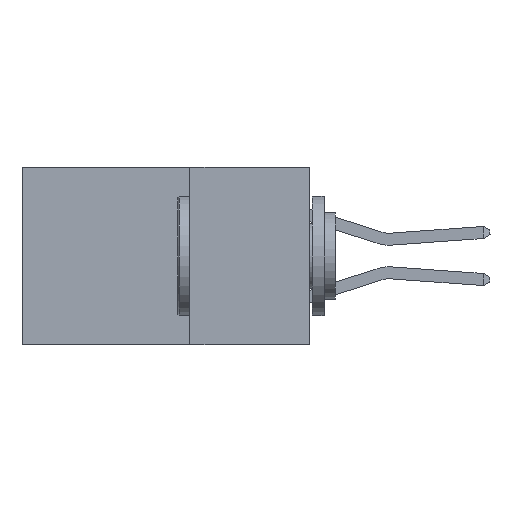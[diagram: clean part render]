
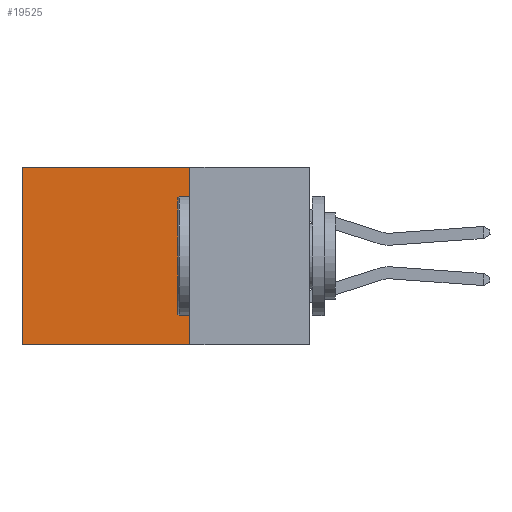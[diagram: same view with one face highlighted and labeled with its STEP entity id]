
A CAD part, left-side view. The second image highlights one B-rep face of the part: STEP entity #19525.
In plain terms, the highlighted planar face has unit normal (-1, 0, 0).
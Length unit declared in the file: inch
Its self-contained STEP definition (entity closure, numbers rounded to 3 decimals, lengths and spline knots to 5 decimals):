
#249 = VERTEX_POINT ( 'NONE', #23125 ) ;
#716 = CARTESIAN_POINT ( 'NONE',  ( 0.2615, 0.6, -0.37 ) ) ;
#1182 = LINE ( 'NONE', #8395, #9789 ) ;
#1190 = CARTESIAN_POINT ( 'NONE',  ( 0.2615, 0.25, -0.37 ) ) ;
#1338 = FACE_OUTER_BOUND ( 'NONE', #1644, .T. ) ;
#1423 = DIRECTION ( 'NONE',  ( 0., 0., -1. ) ) ;
#1644 = EDGE_LOOP ( 'NONE', ( #18930, #4151, #7641, #22586 ) ) ;
#3120 = LINE ( 'NONE', #13941, #11418 ) ;
#3147 = CARTESIAN_POINT ( 'NONE',  ( 0.2615, 0.25, 0. ) ) ;
#4151 = ORIENTED_EDGE ( 'NONE', *, *, #6804, .F. ) ;
#4480 = CARTESIAN_POINT ( 'NONE',  ( 0.2615, 0.6, 0. ) ) ;
#6804 = EDGE_CURVE ( 'NONE', #10332, #18355, #3120, .T. ) ;
#6813 = LINE ( 'NONE', #3147, #8588 ) ;
#7641 = ORIENTED_EDGE ( 'NONE', *, *, #16873, .F. ) ;
#8043 = AXIS2_PLACEMENT_3D ( 'NONE', #8551, #15694, #13925 ) ;
#8395 = CARTESIAN_POINT ( 'NONE',  ( 0.2615, 0.25, -0.37 ) ) ;
#8551 = CARTESIAN_POINT ( 'NONE',  ( 0.2615, 0.25, -0.37 ) ) ;
#8588 = VECTOR ( 'NONE', #19231, 39.37008 ) ;
#9208 = VECTOR ( 'NONE', #12108, 39.37008 ) ;
#9337 = VERTEX_POINT ( 'NONE', #4480 ) ;
#9789 = VECTOR ( 'NONE', #1423, 39.37008 ) ;
#10332 = VERTEX_POINT ( 'NONE', #1190 ) ;
#10803 = LINE ( 'NONE', #17949, #9208 ) ;
#11418 = VECTOR ( 'NONE', #15482, 39.37008 ) ;
#12108 = DIRECTION ( 'NONE',  ( 0., 0., -1. ) ) ;
#13925 = DIRECTION ( 'NONE',  ( 0., 0., -1. ) ) ;
#13941 = CARTESIAN_POINT ( 'NONE',  ( 0.2615, 0.25, -0.37 ) ) ;
#14118 = EDGE_CURVE ( 'NONE', #249, #9337, #6813, .T. ) ;
#15482 = DIRECTION ( 'NONE',  ( 0., 1., 0. ) ) ;
#15694 = DIRECTION ( 'NONE',  ( 1., 0., 0. ) ) ;
#16873 = EDGE_CURVE ( 'NONE', #249, #10332, #1182, .T. ) ;
#17949 = CARTESIAN_POINT ( 'NONE',  ( 0.2615, 0.6, -0.37 ) ) ;
#18355 = VERTEX_POINT ( 'NONE', #716 ) ;
#18930 = ORIENTED_EDGE ( 'NONE', *, *, #20641, .T. ) ;
#19231 = DIRECTION ( 'NONE',  ( 0., 1., 0. ) ) ;
#19525 = ADVANCED_FACE ( 'NONE', ( #1338 ), #22802, .F. ) ;
#20641 = EDGE_CURVE ( 'NONE', #9337, #18355, #10803, .T. ) ;
#22586 = ORIENTED_EDGE ( 'NONE', *, *, #14118, .T. ) ;
#22802 = PLANE ( 'NONE',  #8043 ) ;
#23125 = CARTESIAN_POINT ( 'NONE',  ( 0.2615, 0.25, 0. ) ) ;
